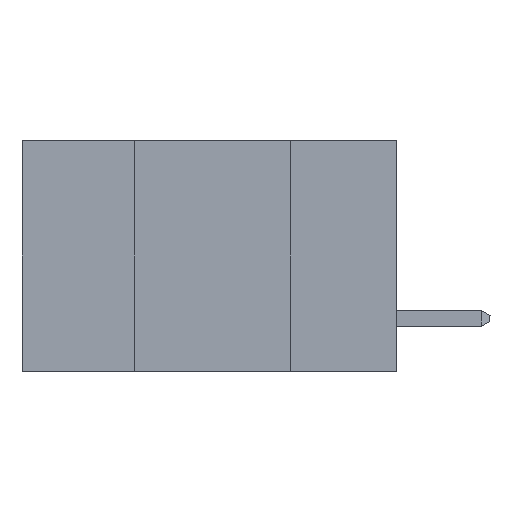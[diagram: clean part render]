
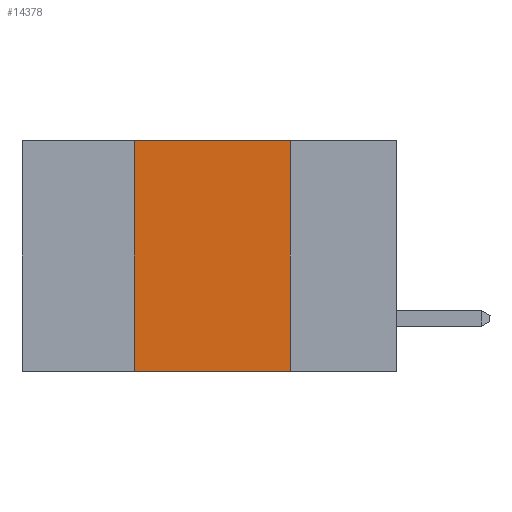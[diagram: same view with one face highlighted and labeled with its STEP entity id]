
A CAD part, left-side view. The second image highlights one B-rep face of the part: STEP entity #14378.
In plain terms, the highlighted planar face has unit normal (-1, 0, 0).
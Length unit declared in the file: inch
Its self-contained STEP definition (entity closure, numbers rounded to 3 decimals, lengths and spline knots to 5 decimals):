
#163 = PLANE ( 'NONE',  #18393 ) ;
#419 = CARTESIAN_POINT ( 'NONE',  ( 0., 0.6, 0. ) ) ;
#600 = VERTEX_POINT ( 'NONE', #25171 ) ;
#894 = DIRECTION ( 'NONE',  ( 0., -1., 0. ) ) ;
#2459 = VECTOR ( 'NONE', #24693, 39.37008 ) ;
#3002 = EDGE_LOOP ( 'NONE', ( #3661, #3783, #11558, #17934 ) ) ;
#3661 = ORIENTED_EDGE ( 'NONE', *, *, #14137, .F. ) ;
#3715 = EDGE_CURVE ( 'NONE', #600, #21941, #11615, .T. ) ;
#3783 = ORIENTED_EDGE ( 'NONE', *, *, #12435, .F. ) ;
#6401 = VECTOR ( 'NONE', #894, 39.37008 ) ;
#7039 = LINE ( 'NONE', #419, #24362 ) ;
#8612 = CARTESIAN_POINT ( 'NONE',  ( 0., 0.17, -0.37 ) ) ;
#9967 = DIRECTION ( 'NONE',  ( 0., 0., -1. ) ) ;
#10067 = DIRECTION ( 'NONE',  ( 0., 0., -1. ) ) ;
#10593 = LINE ( 'NONE', #21714, #12716 ) ;
#11173 = CARTESIAN_POINT ( 'NONE',  ( 0., 0.42, 0. ) ) ;
#11558 = ORIENTED_EDGE ( 'NONE', *, *, #3715, .F. ) ;
#11615 = LINE ( 'NONE', #11173, #2459 ) ;
#12435 = EDGE_CURVE ( 'NONE', #21941, #18330, #7039, .T. ) ;
#12716 = VECTOR ( 'NONE', #10067, 39.37008 ) ;
#13627 = FACE_OUTER_BOUND ( 'NONE', #3002, .T. ) ;
#14070 = DIRECTION ( 'NONE',  ( 0., -1., 0. ) ) ;
#14137 = EDGE_CURVE ( 'NONE', #18330, #23074, #10593, .T. ) ;
#14378 = ADVANCED_FACE ( 'NONE', ( #13627 ), #163, .F. ) ;
#15486 = EDGE_CURVE ( 'NONE', #600, #23074, #23097, .T. ) ;
#15743 = CARTESIAN_POINT ( 'NONE',  ( 0., 0.6, 0. ) ) ;
#17934 = ORIENTED_EDGE ( 'NONE', *, *, #15486, .T. ) ;
#18330 = VERTEX_POINT ( 'NONE', #23824 ) ;
#18393 = AXIS2_PLACEMENT_3D ( 'NONE', #15743, #19633, #9967 ) ;
#19633 = DIRECTION ( 'NONE',  ( 1., 0., 0. ) ) ;
#21335 = CARTESIAN_POINT ( 'NONE',  ( 0., 0.6, -0.37 ) ) ;
#21714 = CARTESIAN_POINT ( 'NONE',  ( 0., 0.17, 0. ) ) ;
#21941 = VERTEX_POINT ( 'NONE', #21961 ) ;
#21961 = CARTESIAN_POINT ( 'NONE',  ( 0., 0.42, 0. ) ) ;
#23074 = VERTEX_POINT ( 'NONE', #8612 ) ;
#23097 = LINE ( 'NONE', #21335, #6401 ) ;
#23824 = CARTESIAN_POINT ( 'NONE',  ( 0., 0.17, 0. ) ) ;
#24362 = VECTOR ( 'NONE', #14070, 39.37008 ) ;
#24693 = DIRECTION ( 'NONE',  ( 0., 0., 1. ) ) ;
#25171 = CARTESIAN_POINT ( 'NONE',  ( 0., 0.42, -0.37 ) ) ;
